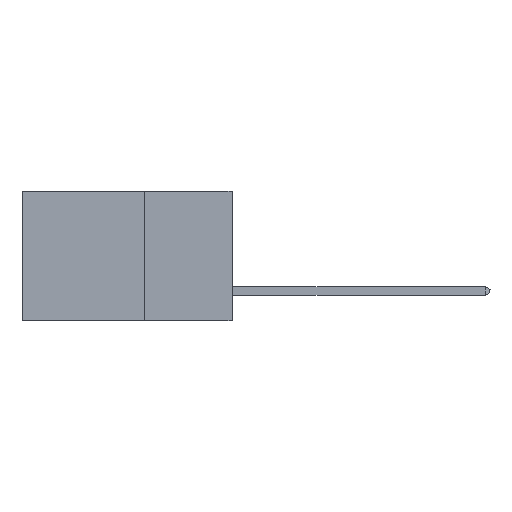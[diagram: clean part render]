
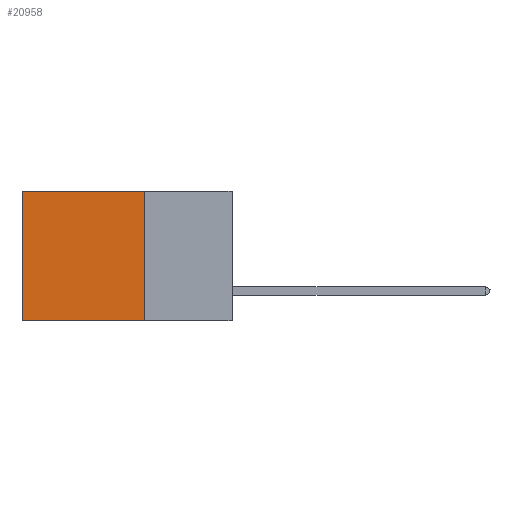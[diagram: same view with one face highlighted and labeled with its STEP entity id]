
A CAD part, left-side view. The second image highlights one B-rep face of the part: STEP entity #20958.
In plain terms, the highlighted planar face has unit normal (-1, 0, 0).
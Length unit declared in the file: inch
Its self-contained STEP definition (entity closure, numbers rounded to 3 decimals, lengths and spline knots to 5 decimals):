
#952 = DIRECTION ( 'NONE',  ( 0., 1., 0. ) ) ;
#992 = DIRECTION ( 'NONE',  ( 0., 0., -1. ) ) ;
#2089 = LINE ( 'NONE', #22586, #31737 ) ;
#3255 = VERTEX_POINT ( 'NONE', #17994 ) ;
#3270 = VERTEX_POINT ( 'NONE', #29614 ) ;
#4590 = DIRECTION ( 'NONE',  ( 0., 1., 0. ) ) ;
#4891 = CARTESIAN_POINT ( 'NONE',  ( 0.2875, 0.25, -0.37 ) ) ;
#5762 = VERTEX_POINT ( 'NONE', #4891 ) ;
#8474 = FACE_OUTER_BOUND ( 'NONE', #29363, .T. ) ;
#9151 = CARTESIAN_POINT ( 'NONE',  ( 0.2875, 0.25, 0. ) ) ;
#9152 = EDGE_CURVE ( 'NONE', #3270, #26987, #9490, .T. ) ;
#9490 = LINE ( 'NONE', #29284, #27519 ) ;
#9826 = EDGE_CURVE ( 'NONE', #3255, #3270, #2089, .T. ) ;
#11383 = ORIENTED_EDGE ( 'NONE', *, *, #18017, .F. ) ;
#11696 = PLANE ( 'NONE',  #18548 ) ;
#12511 = LINE ( 'NONE', #33402, #35300 ) ;
#15191 = ORIENTED_EDGE ( 'NONE', *, *, #9152, .T. ) ;
#17295 = LINE ( 'NONE', #27472, #28318 ) ;
#17994 = CARTESIAN_POINT ( 'NONE',  ( 0.2875, 0.25, 0. ) ) ;
#18017 = EDGE_CURVE ( 'NONE', #5762, #26987, #17295, .T. ) ;
#18231 = ORIENTED_EDGE ( 'NONE', *, *, #18726, .F. ) ;
#18548 = AXIS2_PLACEMENT_3D ( 'NONE', #9151, #38357, #20588 ) ;
#18726 = EDGE_CURVE ( 'NONE', #3255, #5762, #12511, .T. ) ;
#20588 = DIRECTION ( 'NONE',  ( 0., 0., -1. ) ) ;
#20958 = ADVANCED_FACE ( 'NONE', ( #8474 ), #11696, .F. ) ;
#22586 = CARTESIAN_POINT ( 'NONE',  ( 0.2875, 0.25, 0. ) ) ;
#26987 = VERTEX_POINT ( 'NONE', #29735 ) ;
#27472 = CARTESIAN_POINT ( 'NONE',  ( 0.2875, 0.25, -0.37 ) ) ;
#27519 = VECTOR ( 'NONE', #38283, 39.37008 ) ;
#28318 = VECTOR ( 'NONE', #952, 39.37008 ) ;
#28746 = ORIENTED_EDGE ( 'NONE', *, *, #9826, .T. ) ;
#29284 = CARTESIAN_POINT ( 'NONE',  ( 0.2875, 0.6, 0. ) ) ;
#29363 = EDGE_LOOP ( 'NONE', ( #15191, #11383, #18231, #28746 ) ) ;
#29614 = CARTESIAN_POINT ( 'NONE',  ( 0.2875, 0.6, 0. ) ) ;
#29735 = CARTESIAN_POINT ( 'NONE',  ( 0.2875, 0.6, -0.37 ) ) ;
#31737 = VECTOR ( 'NONE', #4590, 39.37008 ) ;
#33402 = CARTESIAN_POINT ( 'NONE',  ( 0.2875, 0.25, 0. ) ) ;
#35300 = VECTOR ( 'NONE', #992, 39.37008 ) ;
#38283 = DIRECTION ( 'NONE',  ( 0., 0., -1. ) ) ;
#38357 = DIRECTION ( 'NONE',  ( 1., 0., 0. ) ) ;
